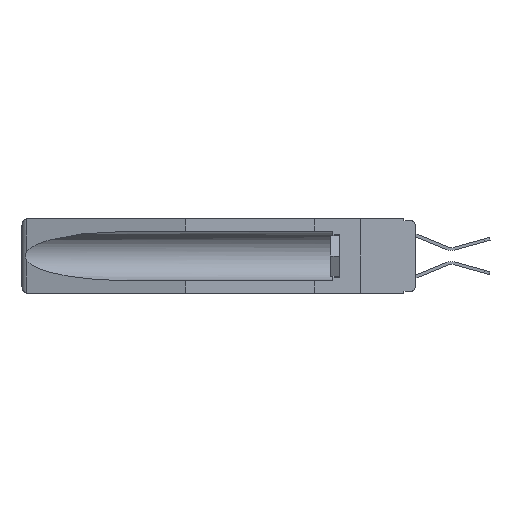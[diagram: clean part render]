
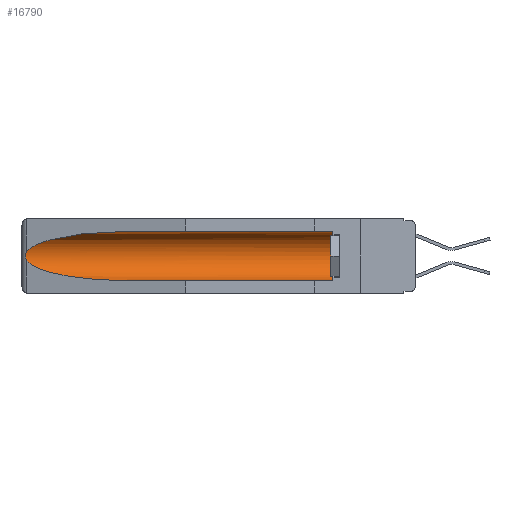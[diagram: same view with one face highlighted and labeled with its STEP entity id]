
A CAD part, left-side view. The second image highlights one B-rep face of the part: STEP entity #16790.
In plain terms, the highlighted cylindrical face has radius 2.857 mm (diameter 5.715 mm), a partial arc.
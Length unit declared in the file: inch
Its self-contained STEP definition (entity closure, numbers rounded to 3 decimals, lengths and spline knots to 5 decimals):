
#133 = CARTESIAN_POINT ( 'NONE',  ( 0.26537, 1.52718, -0.14972 ) ) ;
#348 =( BOUNDED_CURVE ( )  B_SPLINE_CURVE ( 3, ( #8575, #22528, #5121, #13766 ),
 .UNSPECIFIED., .F., .F. ) 
 B_SPLINE_CURVE_WITH_KNOTS ( ( 4, 4 ),
 ( 0.1948, 1.5708 ),
 .UNSPECIFIED. ) 
 CURVE ( )  GEOMETRIC_REPRESENTATION_ITEM ( )  RATIONAL_B_SPLINE_CURVE ( ( 1., 0.848, 0.848, 1. ) ) 
 REPRESENTATION_ITEM ( '' )  );
#1424 = CARTESIAN_POINT ( 'NONE',  ( 0.26537, 1.52718, -0.14972 ) ) ;
#1492 = EDGE_CURVE ( 'NONE', #14391, #8766, #348, .T. ) ;
#1764 = ORIENTED_EDGE ( 'NONE', *, *, #14054, .T. ) ;
#2827 = DIRECTION ( 'NONE',  ( 0., 0., 1. ) ) ;
#2838 = CARTESIAN_POINT ( 'NONE',  ( 0.155, 0.126, -0.284 ) ) ;
#3480 = CARTESIAN_POINT ( 'NONE',  ( 0.21114, 1.30732, -0.059 ) ) ;
#3506 = DIRECTION ( 'NONE',  ( 0., 1., 0. ) ) ;
#3727 = CARTESIAN_POINT ( 'NONE',  ( 0.2673, 1.5327, -0.16383 ) ) ;
#4105 = CYLINDRICAL_SURFACE ( 'NONE', #15789, 0.1125 ) ;
#5002 = CARTESIAN_POINT ( 'NONE',  ( 0.155, 1.07973, -0.284 ) ) ;
#5116 = VECTOR ( 'NONE', #13959, 39.37008 ) ;
#5120 = ORIENTED_EDGE ( 'NONE', *, *, #5655, .T. ) ;
#5121 = CARTESIAN_POINT ( 'NONE',  ( 0.21114, 1.30732, -0.284 ) ) ;
#5141 = VERTEX_POINT ( 'NONE', #1424 ) ;
#5251 = LINE ( 'NONE', #12382, #22638 ) ;
#5319 = EDGE_CURVE ( 'NONE', #6385, #8766, #5251, .T. ) ;
#5655 = EDGE_CURVE ( 'NONE', #6385, #19779, #8167, .T. ) ;
#6385 = VERTEX_POINT ( 'NONE', #2838 ) ;
#6830 = CARTESIAN_POINT ( 'NONE',  ( 0.155, 1.07973, -0.059 ) ) ;
#6974 = VERTEX_POINT ( 'NONE', #20802 ) ;
#7421 = CARTESIAN_POINT ( 'NONE',  ( 0.2675, 1.53308, -0.16763 ) ) ;
#8167 = CIRCLE ( 'NONE', #21304, 0.1125 ) ;
#8338 = ORIENTED_EDGE ( 'NONE', *, *, #8504, .T. ) ;
#8504 = EDGE_CURVE ( 'NONE', #5141, #14391, #17152, .T. ) ;
#8575 = CARTESIAN_POINT ( 'NONE',  ( 0.26537, 1.52718, -0.19328 ) ) ;
#8766 = VERTEX_POINT ( 'NONE', #5002 ) ;
#9076 = CARTESIAN_POINT ( 'NONE',  ( 0.26597, 1.52961, -0.15275 ) ) ;
#9094 =( BOUNDED_CURVE ( )  B_SPLINE_CURVE ( 3, ( #6830, #3480, #13994, #22995 ),
 .UNSPECIFIED., .F., .F. ) 
 B_SPLINE_CURVE_WITH_KNOTS ( ( 4, 4 ),
 ( 4.71239, 6.08839 ),
 .UNSPECIFIED. ) 
 CURVE ( )  GEOMETRIC_REPRESENTATION_ITEM ( )  RATIONAL_B_SPLINE_CURVE ( ( 1., 0.848, 0.848, 1. ) ) 
 REPRESENTATION_ITEM ( '' )  );
#9798 = DIRECTION ( 'NONE',  ( 0., 0., 1. ) ) ;
#10123 = DIRECTION ( 'NONE',  ( 0., -1., 0. ) ) ;
#12082 = CARTESIAN_POINT ( 'NONE',  ( 0.155, -0.30754, -0.059 ) ) ;
#12382 = CARTESIAN_POINT ( 'NONE',  ( 0.155, -0.30754, -0.284 ) ) ;
#13766 = CARTESIAN_POINT ( 'NONE',  ( 0.155, 1.07973, -0.284 ) ) ;
#13959 = DIRECTION ( 'NONE',  ( 0., 1., 0. ) ) ;
#13994 = CARTESIAN_POINT ( 'NONE',  ( 0.25451, 1.48313, -0.09465 ) ) ;
#14054 = EDGE_CURVE ( 'NONE', #19779, #6974, #17346, .T. ) ;
#14181 = ORIENTED_EDGE ( 'NONE', *, *, #18444, .T. ) ;
#14248 = CARTESIAN_POINT ( 'NONE',  ( 0.2673, 1.53269, -0.17917 ) ) ;
#14344 = CARTESIAN_POINT ( 'NONE',  ( 0.26537, 1.52718, -0.19328 ) ) ;
#14391 = VERTEX_POINT ( 'NONE', #14344 ) ;
#14598 = CARTESIAN_POINT ( 'NONE',  ( 0.26655, 1.53094, -0.18657 ) ) ;
#14714 = CARTESIAN_POINT ( 'NONE',  ( 0.26654, 1.53092, -0.15636 ) ) ;
#14971 = CARTESIAN_POINT ( 'NONE',  ( 0.155, -0.30754, -0.1715 ) ) ;
#15560 = ORIENTED_EDGE ( 'NONE', *, *, #1492, .T. ) ;
#15785 = ORIENTED_EDGE ( 'NONE', *, *, #5319, .F. ) ;
#15789 = AXIS2_PLACEMENT_3D ( 'NONE', #14971, #22114, #2827 ) ;
#16569 = CARTESIAN_POINT ( 'NONE',  ( 0.2675, 1.53308, -0.17534 ) ) ;
#16790 = ADVANCED_FACE ( 'NONE', ( #21892 ), #4105, .F. ) ;
#17152 = B_SPLINE_CURVE_WITH_KNOTS ( 'NONE', 3,
 ( #133, #9076, #14714, #3727, #7421, #16569, #14248, #14598, #21399, #19975 ),
 .UNSPECIFIED., .F., .F.,
 ( 4, 2, 2, 2, 4 ),
 ( 0., 0.00029, 0.00058, 0.00087, 0.00117 ),
 .UNSPECIFIED. ) ;
#17346 = LINE ( 'NONE', #12082, #5116 ) ;
#18286 = EDGE_LOOP ( 'NONE', ( #14181, #8338, #15560, #15785, #5120, #1764 ) ) ;
#18444 = EDGE_CURVE ( 'NONE', #6974, #5141, #9094, .T. ) ;
#19779 = VERTEX_POINT ( 'NONE', #20668 ) ;
#19975 = CARTESIAN_POINT ( 'NONE',  ( 0.26537, 1.52718, -0.19328 ) ) ;
#20448 = CARTESIAN_POINT ( 'NONE',  ( 0.155, 0.126, -0.1715 ) ) ;
#20668 = CARTESIAN_POINT ( 'NONE',  ( 0.155, 0.126, -0.059 ) ) ;
#20802 = CARTESIAN_POINT ( 'NONE',  ( 0.155, 1.07973, -0.059 ) ) ;
#21304 = AXIS2_PLACEMENT_3D ( 'NONE', #20448, #10123, #9798 ) ;
#21399 = CARTESIAN_POINT ( 'NONE',  ( 0.26597, 1.5296, -0.19026 ) ) ;
#21892 = FACE_OUTER_BOUND ( 'NONE', #18286, .T. ) ;
#22114 = DIRECTION ( 'NONE',  ( 0., 1., 0. ) ) ;
#22528 = CARTESIAN_POINT ( 'NONE',  ( 0.25451, 1.48313, -0.24835 ) ) ;
#22638 = VECTOR ( 'NONE', #3506, 39.37008 ) ;
#22995 = CARTESIAN_POINT ( 'NONE',  ( 0.26537, 1.52718, -0.14972 ) ) ;
